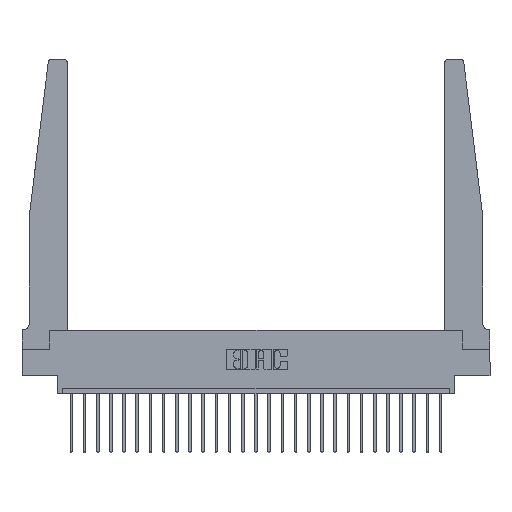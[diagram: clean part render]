
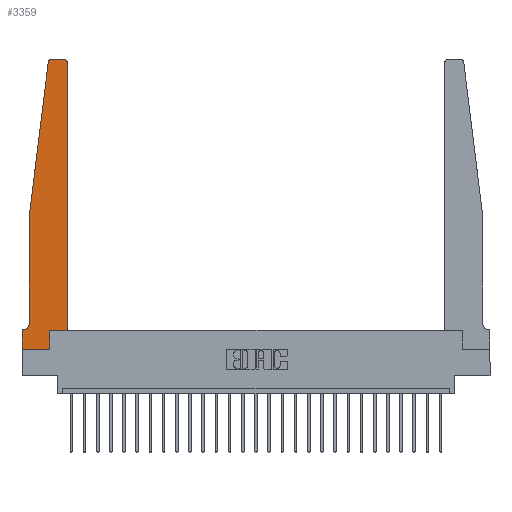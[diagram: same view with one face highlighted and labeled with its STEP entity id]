
A CAD part, top view. The second image highlights one B-rep face of the part: STEP entity #3359.
In plain terms, the highlighted planar face has unit normal (0, 0, 1).
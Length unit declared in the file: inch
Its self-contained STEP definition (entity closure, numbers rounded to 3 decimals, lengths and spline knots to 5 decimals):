
#731 = VERTEX_POINT ( 'NONE', #8184 ) ;
#776 = EDGE_CURVE ( 'NONE', #15475, #1427, #13572, .T. ) ;
#1262 = ORIENTED_EDGE ( 'NONE', *, *, #5324, .T. ) ;
#1345 = DIRECTION ( 'NONE',  ( 1., 0., 0. ) ) ;
#1427 = VERTEX_POINT ( 'NONE', #18450 ) ;
#1580 = LINE ( 'NONE', #7044, #3607 ) ;
#1682 = VECTOR ( 'NONE', #13756, 39.37008 ) ;
#1781 = DIRECTION ( 'NONE',  ( 0., 0., 1. ) ) ;
#2395 = CARTESIAN_POINT ( 'NONE',  ( 0.25, 2.75, 0.37 ) ) ;
#3023 = EDGE_CURVE ( 'NONE', #13409, #9271, #3095, .T. ) ;
#3056 = CARTESIAN_POINT ( 'NONE',  ( 0.27653, 2.75, 0.37 ) ) ;
#3095 = LINE ( 'NONE', #24045, #14333 ) ;
#3111 = CARTESIAN_POINT ( 'NONE',  ( 0.425, 0.18, 0.37 ) ) ;
#3193 = CARTESIAN_POINT ( 'NONE',  ( 0.425, 0.18, 0.37 ) ) ;
#3359 = ADVANCED_FACE ( 'NONE', ( #7598 ), #20911, .T. ) ;
#3607 = VECTOR ( 'NONE', #1345, 39.37008 ) ;
#3801 = CARTESIAN_POINT ( 'NONE',  ( 0., 0.1875, 0.37 ) ) ;
#4302 = CARTESIAN_POINT ( 'NONE',  ( 0.2605, 0.18, 0.37 ) ) ;
#4385 = CARTESIAN_POINT ( 'NONE',  ( 0.065, 1.25, 0.37 ) ) ;
#4649 = EDGE_CURVE ( 'NONE', #5418, #15567, #22112, .T. ) ;
#4762 = VECTOR ( 'NONE', #8662, 39.37008 ) ;
#5204 = DIRECTION ( 'NONE',  ( 1., 0., 0. ) ) ;
#5318 = ORIENTED_EDGE ( 'NONE', *, *, #9199, .T. ) ;
#5324 = EDGE_CURVE ( 'NONE', #21707, #15475, #22030, .T. ) ;
#5418 = VERTEX_POINT ( 'NONE', #3111 ) ;
#5476 = CARTESIAN_POINT ( 'NONE',  ( 0., 0., 0.37 ) ) ;
#5620 = ORIENTED_EDGE ( 'NONE', *, *, #9906, .T. ) ;
#5797 = ORIENTED_EDGE ( 'NONE', *, *, #19488, .T. ) ;
#5835 = DIRECTION ( 'NONE',  ( 0., 1., 0. ) ) ;
#6097 = ORIENTED_EDGE ( 'NONE', *, *, #14978, .T. ) ;
#6520 = CIRCLE ( 'NONE', #6928, 0.03 ) ;
#6556 = CARTESIAN_POINT ( 'NONE',  ( 0.24675, 2.72367, 0.37 ) ) ;
#6928 = AXIS2_PLACEMENT_3D ( 'NONE', #12807, #9013, #5204 ) ;
#7044 = CARTESIAN_POINT ( 'NONE',  ( 0.425, 0.18, 0.37 ) ) ;
#7598 = FACE_OUTER_BOUND ( 'NONE', #11186, .T. ) ;
#8184 = CARTESIAN_POINT ( 'NONE',  ( 0.2605, 0.18, 0.37 ) ) ;
#8235 = VECTOR ( 'NONE', #24648, 39.37008 ) ;
#8504 = CARTESIAN_POINT ( 'NONE',  ( 0.065, 0.2375, 0.37 ) ) ;
#8612 = LINE ( 'NONE', #2395, #14982 ) ;
#8662 = DIRECTION ( 'NONE',  ( -1., 0., 0. ) ) ;
#8977 = CIRCLE ( 'NONE', #21124, 0.03 ) ;
#9013 = DIRECTION ( 'NONE',  ( 0., 0., 1. ) ) ;
#9199 = EDGE_CURVE ( 'NONE', #9271, #12095, #11576, .T. ) ;
#9271 = VERTEX_POINT ( 'NONE', #23870 ) ;
#9346 = VECTOR ( 'NONE', #10928, 39.37008 ) ;
#9423 = ORIENTED_EDGE ( 'NONE', *, *, #4649, .T. ) ;
#9661 = ORIENTED_EDGE ( 'NONE', *, *, #21893, .T. ) ;
#9906 = EDGE_CURVE ( 'NONE', #731, #5418, #1580, .T. ) ;
#10057 = CARTESIAN_POINT ( 'NONE',  ( 0.065, 1.25, 0.37 ) ) ;
#10117 = DIRECTION ( 'NONE',  ( -1., 0., 0. ) ) ;
#10822 = DIRECTION ( 'NONE',  ( 0., -1., 0. ) ) ;
#10928 = DIRECTION ( 'NONE',  ( 0., 1., 0. ) ) ;
#11186 = EDGE_LOOP ( 'NONE', ( #11471, #13028, #5797, #1262, #19612, #6097, #21899, #5318, #9661, #5620, #9423, #21725 ) ) ;
#11471 = ORIENTED_EDGE ( 'NONE', *, *, #20813, .T. ) ;
#11576 = LINE ( 'NONE', #5476, #8235 ) ;
#12087 = CARTESIAN_POINT ( 'NONE',  ( 0.065, 0.1875, 0.37 ) ) ;
#12095 = VERTEX_POINT ( 'NONE', #22704 ) ;
#12807 = CARTESIAN_POINT ( 'NONE',  ( 0.27653, 2.72, 0.37 ) ) ;
#13028 = ORIENTED_EDGE ( 'NONE', *, *, #24669, .T. ) ;
#13383 = VECTOR ( 'NONE', #14033, 39.37008 ) ;
#13409 = VERTEX_POINT ( 'NONE', #14757 ) ;
#13572 = CIRCLE ( 'NONE', #19254, 0.05 ) ;
#13756 = DIRECTION ( 'NONE',  ( 0., -1., 0. ) ) ;
#14033 = DIRECTION ( 'NONE',  ( -0.122, -0.992, 0. ) ) ;
#14333 = VECTOR ( 'NONE', #10822, 39.37008 ) ;
#14757 = CARTESIAN_POINT ( 'NONE',  ( 0., 0.1875, 0.37 ) ) ;
#14978 = EDGE_CURVE ( 'NONE', #1427, #13409, #16007, .T. ) ;
#14982 = VECTOR ( 'NONE', #10117, 39.37008 ) ;
#15055 = CARTESIAN_POINT ( 'NONE',  ( 0.395, 2.72, 0.37 ) ) ;
#15077 = CARTESIAN_POINT ( 'NONE',  ( 0.015, 0.2375, 0.37 ) ) ;
#15475 = VERTEX_POINT ( 'NONE', #8504 ) ;
#15539 = VERTEX_POINT ( 'NONE', #6556 ) ;
#15567 = VERTEX_POINT ( 'NONE', #17707 ) ;
#16007 = LINE ( 'NONE', #12087, #4762 ) ;
#17482 = LINE ( 'NONE', #4302, #21521 ) ;
#17707 = CARTESIAN_POINT ( 'NONE',  ( 0.425, 2.72, 0.37 ) ) ;
#18450 = CARTESIAN_POINT ( 'NONE',  ( 0.015, 0.1875, 0.37 ) ) ;
#19005 = DIRECTION ( 'NONE',  ( -1., 0., 0. ) ) ;
#19254 = AXIS2_PLACEMENT_3D ( 'NONE', #15077, #22830, #19005 ) ;
#19488 = EDGE_CURVE ( 'NONE', #15539, #21707, #23833, .T. ) ;
#19612 = ORIENTED_EDGE ( 'NONE', *, *, #776, .T. ) ;
#20137 = VERTEX_POINT ( 'NONE', #22852 ) ;
#20395 = VERTEX_POINT ( 'NONE', #3056 ) ;
#20660 = DIRECTION ( 'NONE',  ( 1., 0., 0. ) ) ;
#20813 = EDGE_CURVE ( 'NONE', #20137, #20395, #8612, .T. ) ;
#20911 = PLANE ( 'NONE',  #24722 ) ;
#21124 = AXIS2_PLACEMENT_3D ( 'NONE', #15055, #24599, #22812 ) ;
#21521 = VECTOR ( 'NONE', #5835, 39.37008 ) ;
#21707 = VERTEX_POINT ( 'NONE', #10057 ) ;
#21725 = ORIENTED_EDGE ( 'NONE', *, *, #24997, .T. ) ;
#21893 = EDGE_CURVE ( 'NONE', #12095, #731, #17482, .T. ) ;
#21899 = ORIENTED_EDGE ( 'NONE', *, *, #3023, .T. ) ;
#22030 = LINE ( 'NONE', #4385, #1682 ) ;
#22054 = CARTESIAN_POINT ( 'NONE',  ( 0.065, 1.25, 0.37 ) ) ;
#22112 = LINE ( 'NONE', #3193, #9346 ) ;
#22704 = CARTESIAN_POINT ( 'NONE',  ( 0.2605, 0., 0.37 ) ) ;
#22812 = DIRECTION ( 'NONE',  ( 1., 0., 0. ) ) ;
#22830 = DIRECTION ( 'NONE',  ( 0., 0., -1. ) ) ;
#22852 = CARTESIAN_POINT ( 'NONE',  ( 0.395, 2.75, 0.37 ) ) ;
#23833 = LINE ( 'NONE', #22054, #13383 ) ;
#23870 = CARTESIAN_POINT ( 'NONE',  ( 0., 0., 0.37 ) ) ;
#24045 = CARTESIAN_POINT ( 'NONE',  ( 0., 0., 0.37 ) ) ;
#24599 = DIRECTION ( 'NONE',  ( 0., 0., 1. ) ) ;
#24648 = DIRECTION ( 'NONE',  ( 1., 0., 0. ) ) ;
#24669 = EDGE_CURVE ( 'NONE', #20395, #15539, #6520, .T. ) ;
#24722 = AXIS2_PLACEMENT_3D ( 'NONE', #3801, #1781, #20660 ) ;
#24997 = EDGE_CURVE ( 'NONE', #15567, #20137, #8977, .T. ) ;
